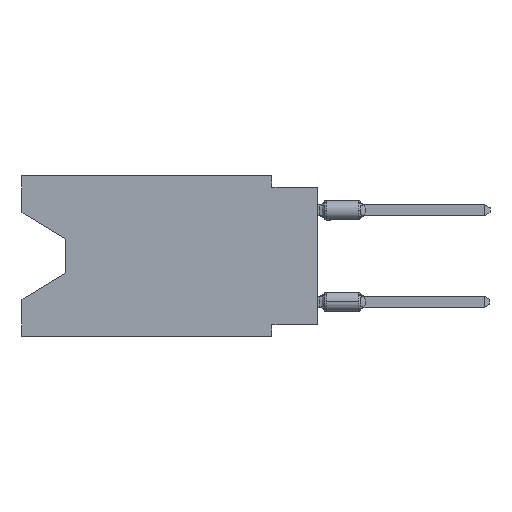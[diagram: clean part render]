
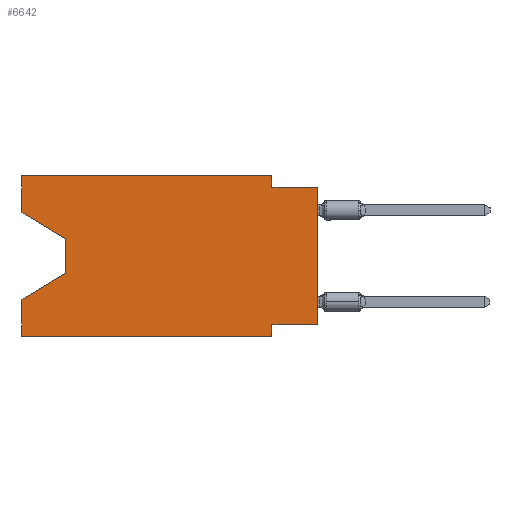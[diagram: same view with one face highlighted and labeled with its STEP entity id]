
A CAD part, left-side view. The second image highlights one B-rep face of the part: STEP entity #6642.
In plain terms, the highlighted planar face has unit normal (-1, 0, 0).
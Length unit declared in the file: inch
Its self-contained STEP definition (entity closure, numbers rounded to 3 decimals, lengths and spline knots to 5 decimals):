
#677 = CARTESIAN_POINT ( 'NONE',  ( 0., 0., -0.025 ) ) ;
#862 = LINE ( 'NONE', #53254, #41573 ) ;
#884 = LINE ( 'NONE', #31070, #4948 ) ;
#1324 = DIRECTION ( 'NONE',  ( 0., 0.855, -0.519 ) ) ;
#1534 = DIRECTION ( 'NONE',  ( 0., 0., -1. ) ) ;
#2190 = DIRECTION ( 'NONE',  ( 0., 1., 0. ) ) ;
#3717 = EDGE_CURVE ( 'NONE', #47100, #48118, #22046, .T. ) ;
#4258 = EDGE_CURVE ( 'NONE', #37047, #55167, #13176, .T. ) ;
#4315 = CARTESIAN_POINT ( 'NONE',  ( 0., 0.55, -0.212 ) ) ;
#4948 = VECTOR ( 'NONE', #10270, 39.37008 ) ;
#5174 = EDGE_CURVE ( 'NONE', #37047, #22635, #20100, .T. ) ;
#5843 = VECTOR ( 'NONE', #1534, 39.37008 ) ;
#6642 = ADVANCED_FACE ( 'NONE', ( #49149 ), #15285, .F. ) ;
#7236 = ORIENTED_EDGE ( 'NONE', *, *, #28130, .F. ) ;
#9967 = CARTESIAN_POINT ( 'NONE',  ( 0., 0.1, 0. ) ) ;
#10270 = DIRECTION ( 'NONE',  ( 0., 0., 1. ) ) ;
#10347 = CARTESIAN_POINT ( 'NONE',  ( 0., 0.1, -0.35 ) ) ;
#10440 = DIRECTION ( 'NONE',  ( 0., 0., -1. ) ) ;
#10484 = VECTOR ( 'NONE', #47963, 39.37008 ) ;
#10830 = CARTESIAN_POINT ( 'NONE',  ( 0., 0., -0.325 ) ) ;
#10904 = CARTESIAN_POINT ( 'NONE',  ( 0., 0.645, -0.08025 ) ) ;
#11011 = LINE ( 'NONE', #40337, #26882 ) ;
#11918 = CARTESIAN_POINT ( 'NONE',  ( 0., 0.1, -0.325 ) ) ;
#12090 = VERTEX_POINT ( 'NONE', #11918 ) ;
#12310 = CARTESIAN_POINT ( 'NONE',  ( 0., 0.1, 0. ) ) ;
#13176 = LINE ( 'NONE', #30527, #47506 ) ;
#15173 = VERTEX_POINT ( 'NONE', #46000 ) ;
#15285 = PLANE ( 'NONE',  #45438 ) ;
#15337 = LINE ( 'NONE', #53213, #15451 ) ;
#15451 = VECTOR ( 'NONE', #32441, 39.37008 ) ;
#15905 = LINE ( 'NONE', #54892, #21847 ) ;
#16353 = EDGE_CURVE ( 'NONE', #12090, #15173, #32573, .T. ) ;
#16813 = EDGE_CURVE ( 'NONE', #42618, #22384, #884, .T. ) ;
#16816 = ORIENTED_EDGE ( 'NONE', *, *, #56027, .T. ) ;
#19902 = ORIENTED_EDGE ( 'NONE', *, *, #5174, .T. ) ;
#20100 = LINE ( 'NONE', #49426, #20150 ) ;
#20150 = VECTOR ( 'NONE', #28644, 39.37008 ) ;
#21847 = VECTOR ( 'NONE', #33278, 39.37008 ) ;
#21979 = EDGE_LOOP ( 'NONE', ( #19902, #38681, #29512, #38154, #16816, #43646, #7236, #46960, #50756, #44289, #50683, #28979 ) ) ;
#22046 = LINE ( 'NONE', #677, #10484 ) ;
#22384 = VERTEX_POINT ( 'NONE', #23162 ) ;
#22635 = VERTEX_POINT ( 'NONE', #26237 ) ;
#23162 = CARTESIAN_POINT ( 'NONE',  ( 0., 0.645, -0.26975 ) ) ;
#24192 = VERTEX_POINT ( 'NONE', #9967 ) ;
#25953 = DIRECTION ( 'NONE',  ( 0., -1., 0. ) ) ;
#26237 = CARTESIAN_POINT ( 'NONE',  ( 0., 0.55, -0.138 ) ) ;
#26803 = EDGE_CURVE ( 'NONE', #55167, #24192, #862, .T. ) ;
#26882 = VECTOR ( 'NONE', #2190, 39.37008 ) ;
#28130 = EDGE_CURVE ( 'NONE', #54601, #12090, #11011, .T. ) ;
#28493 = VECTOR ( 'NONE', #38406, 39.37008 ) ;
#28644 = DIRECTION ( 'NONE',  ( 0., -0.855, -0.519 ) ) ;
#28979 = ORIENTED_EDGE ( 'NONE', *, *, #4258, .F. ) ;
#29512 = ORIENTED_EDGE ( 'NONE', *, *, #56206, .T. ) ;
#30277 = EDGE_CURVE ( 'NONE', #24192, #47100, #46167, .T. ) ;
#30527 = CARTESIAN_POINT ( 'NONE',  ( 0., 0.645, 0. ) ) ;
#31070 = CARTESIAN_POINT ( 'NONE',  ( 0., 0.645, 0. ) ) ;
#32441 = DIRECTION ( 'NONE',  ( 0., 0., 1. ) ) ;
#32508 = VECTOR ( 'NONE', #34226, 39.37008 ) ;
#32573 = LINE ( 'NONE', #10347, #5843 ) ;
#32924 = DIRECTION ( 'NONE',  ( 1., 0., 0. ) ) ;
#33278 = DIRECTION ( 'NONE',  ( 0., -1., 0. ) ) ;
#34226 = DIRECTION ( 'NONE',  ( 0., 0., -1. ) ) ;
#36339 = CARTESIAN_POINT ( 'NONE',  ( 0., 0.55, -0.212 ) ) ;
#37047 = VERTEX_POINT ( 'NONE', #10904 ) ;
#38154 = ORIENTED_EDGE ( 'NONE', *, *, #16813, .F. ) ;
#38406 = DIRECTION ( 'NONE',  ( 0., 0., -1. ) ) ;
#38681 = ORIENTED_EDGE ( 'NONE', *, *, #44892, .T. ) ;
#40337 = CARTESIAN_POINT ( 'NONE',  ( 0., 0., -0.325 ) ) ;
#41573 = VECTOR ( 'NONE', #25953, 39.37008 ) ;
#42523 = CARTESIAN_POINT ( 'NONE',  ( 0., 0., -0.025 ) ) ;
#42618 = VERTEX_POINT ( 'NONE', #50524 ) ;
#43646 = ORIENTED_EDGE ( 'NONE', *, *, #16353, .F. ) ;
#44289 = ORIENTED_EDGE ( 'NONE', *, *, #30277, .F. ) ;
#44604 = VERTEX_POINT ( 'NONE', #4315 ) ;
#44892 = EDGE_CURVE ( 'NONE', #22635, #44604, #54924, .T. ) ;
#45174 = CARTESIAN_POINT ( 'NONE',  ( 0., 0.645, 0. ) ) ;
#45438 = AXIS2_PLACEMENT_3D ( 'NONE', #45174, #32924, #10440 ) ;
#46000 = CARTESIAN_POINT ( 'NONE',  ( 0., 0.1, -0.35 ) ) ;
#46167 = LINE ( 'NONE', #12310, #32508 ) ;
#46960 = ORIENTED_EDGE ( 'NONE', *, *, #55854, .T. ) ;
#47100 = VERTEX_POINT ( 'NONE', #49018 ) ;
#47506 = VECTOR ( 'NONE', #47897, 39.37008 ) ;
#47897 = DIRECTION ( 'NONE',  ( 0., 0., 1. ) ) ;
#47963 = DIRECTION ( 'NONE',  ( 0., -1., 0. ) ) ;
#48118 = VERTEX_POINT ( 'NONE', #42523 ) ;
#48593 = LINE ( 'NONE', #36339, #49085 ) ;
#49018 = CARTESIAN_POINT ( 'NONE',  ( 0., 0.1, -0.025 ) ) ;
#49085 = VECTOR ( 'NONE', #1324, 39.37008 ) ;
#49149 = FACE_OUTER_BOUND ( 'NONE', #21979, .T. ) ;
#49426 = CARTESIAN_POINT ( 'NONE',  ( 0., 0.645, -0.08025 ) ) ;
#50524 = CARTESIAN_POINT ( 'NONE',  ( 0., 0.645, -0.35 ) ) ;
#50683 = ORIENTED_EDGE ( 'NONE', *, *, #26803, .F. ) ;
#50756 = ORIENTED_EDGE ( 'NONE', *, *, #3717, .F. ) ;
#50930 = CARTESIAN_POINT ( 'NONE',  ( 0., 0.55, -0.138 ) ) ;
#53213 = CARTESIAN_POINT ( 'NONE',  ( 0., 0., 0. ) ) ;
#53254 = CARTESIAN_POINT ( 'NONE',  ( 0., 0.645, 0. ) ) ;
#54601 = VERTEX_POINT ( 'NONE', #10830 ) ;
#54892 = CARTESIAN_POINT ( 'NONE',  ( 0., 0.645, -0.35 ) ) ;
#54924 = LINE ( 'NONE', #50930, #28493 ) ;
#55167 = VERTEX_POINT ( 'NONE', #55735 ) ;
#55735 = CARTESIAN_POINT ( 'NONE',  ( 0., 0.645, 0. ) ) ;
#55854 = EDGE_CURVE ( 'NONE', #54601, #48118, #15337, .T. ) ;
#56027 = EDGE_CURVE ( 'NONE', #42618, #15173, #15905, .T. ) ;
#56206 = EDGE_CURVE ( 'NONE', #44604, #22384, #48593, .T. ) ;
